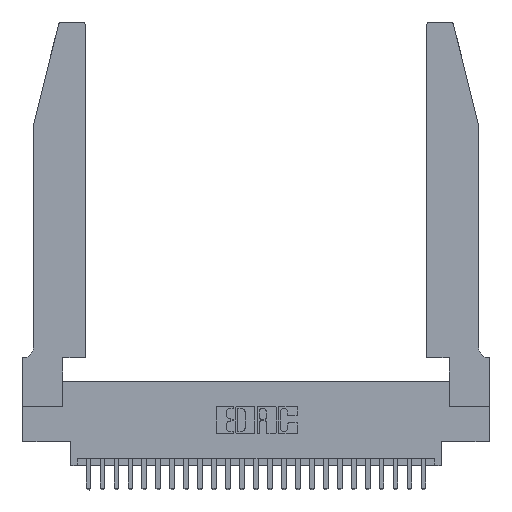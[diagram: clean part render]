
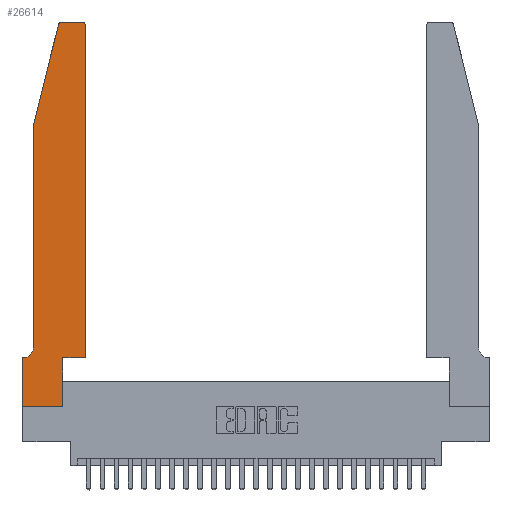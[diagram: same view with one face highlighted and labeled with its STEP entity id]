
A CAD part, top view. The second image highlights one B-rep face of the part: STEP entity #26614.
In plain terms, the highlighted planar face has unit normal (0, 0, 1).
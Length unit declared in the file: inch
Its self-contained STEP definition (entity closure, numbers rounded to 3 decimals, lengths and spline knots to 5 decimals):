
#441 = DIRECTION ( 'NONE',  ( 0., 1., 0. ) ) ;
#812 = ORIENTED_EDGE ( 'NONE', *, *, #13070, .T. ) ;
#826 = CARTESIAN_POINT ( 'NONE',  ( 0.4505, 0.35, 0.37 ) ) ;
#1180 = CIRCLE ( 'NONE', #20505, 0.07 ) ;
#1623 = DIRECTION ( 'NONE',  ( -0.239, -0.971, 0. ) ) ;
#1858 = EDGE_CURVE ( 'NONE', #19033, #4692, #2163, .T. ) ;
#2163 = LINE ( 'NONE', #8192, #22024 ) ;
#2244 = DIRECTION ( 'NONE',  ( 0., 0., 1. ) ) ;
#3155 = DIRECTION ( 'NONE',  ( 1., 0., 0. ) ) ;
#3374 = CARTESIAN_POINT ( 'NONE',  ( 0., 0.35, 0.37 ) ) ;
#3847 = ORIENTED_EDGE ( 'NONE', *, *, #15759, .T. ) ;
#3925 = EDGE_CURVE ( 'NONE', #5902, #19767, #11113, .T. ) ;
#4187 = CARTESIAN_POINT ( 'NONE',  ( 0.4505, 0.35, 0.37 ) ) ;
#4507 = VECTOR ( 'NONE', #7027, 39.37008 ) ;
#4586 = CARTESIAN_POINT ( 'NONE',  ( 0.2865, 0.35, 0.37 ) ) ;
#4692 = VERTEX_POINT ( 'NONE', #15383 ) ;
#5426 = CARTESIAN_POINT ( 'NONE',  ( 0., 0.35, 0.37 ) ) ;
#5545 = VERTEX_POINT ( 'NONE', #8538 ) ;
#5902 = VERTEX_POINT ( 'NONE', #25741 ) ;
#6135 = ORIENTED_EDGE ( 'NONE', *, *, #3925, .T. ) ;
#6289 = CARTESIAN_POINT ( 'NONE',  ( 0.284, 2.72, 0.37 ) ) ;
#6410 = EDGE_CURVE ( 'NONE', #12512, #19033, #11972, .T. ) ;
#6717 = VECTOR ( 'NONE', #21483, 39.37008 ) ;
#7027 = DIRECTION ( 'NONE',  ( 1., 0., 0. ) ) ;
#7376 = CIRCLE ( 'NONE', #15077, 0.03 ) ;
#7941 = CARTESIAN_POINT ( 'NONE',  ( 0.0755, 2., 0.37 ) ) ;
#7953 = VERTEX_POINT ( 'NONE', #15384 ) ;
#7997 = LINE ( 'NONE', #7941, #19749 ) ;
#8192 = CARTESIAN_POINT ( 'NONE',  ( 0., 0., 0.37 ) ) ;
#8538 = CARTESIAN_POINT ( 'NONE',  ( 0.4505, 2.72, 0.37 ) ) ;
#8663 = DIRECTION ( 'NONE',  ( 0., 0., -1. ) ) ;
#8692 = VECTOR ( 'NONE', #3155, 39.37008 ) ;
#9043 = VECTOR ( 'NONE', #12936, 39.37008 ) ;
#9156 = FACE_OUTER_BOUND ( 'NONE', #16446, .T. ) ;
#9232 = ORIENTED_EDGE ( 'NONE', *, *, #6410, .T. ) ;
#9514 = VERTEX_POINT ( 'NONE', #9903 ) ;
#9901 = ORIENTED_EDGE ( 'NONE', *, *, #1858, .T. ) ;
#9903 = CARTESIAN_POINT ( 'NONE',  ( 0.2865, 0., 0.37 ) ) ;
#10303 = DIRECTION ( 'NONE',  ( 0., -1., 0. ) ) ;
#10632 = VERTEX_POINT ( 'NONE', #23169 ) ;
#10888 = EDGE_CURVE ( 'NONE', #9514, #26902, #20522, .T. ) ;
#10955 = CARTESIAN_POINT ( 'NONE',  ( 0.2605, 2.75, 0.37 ) ) ;
#11060 = VECTOR ( 'NONE', #441, 39.37008 ) ;
#11113 = LINE ( 'NONE', #10955, #12097 ) ;
#11406 = ORIENTED_EDGE ( 'NONE', *, *, #16153, .T. ) ;
#11458 = VERTEX_POINT ( 'NONE', #21474 ) ;
#11972 = LINE ( 'NONE', #23353, #9043 ) ;
#11974 = LINE ( 'NONE', #21814, #8692 ) ;
#12097 = VECTOR ( 'NONE', #21168, 39.37008 ) ;
#12181 = EDGE_CURVE ( 'NONE', #10632, #11458, #21130, .T. ) ;
#12512 = VERTEX_POINT ( 'NONE', #17127 ) ;
#12936 = DIRECTION ( 'NONE',  ( -1., 0., 0. ) ) ;
#13070 = EDGE_CURVE ( 'NONE', #20444, #5545, #23710, .T. ) ;
#13475 = EDGE_CURVE ( 'NONE', #11458, #7953, #7997, .T. ) ;
#13948 = DIRECTION ( 'NONE',  ( 0., 0., 1. ) ) ;
#14024 = CARTESIAN_POINT ( 'NONE',  ( 0.0755, 2., 0.37 ) ) ;
#14582 = CIRCLE ( 'NONE', #26066, 0.03 ) ;
#14740 = DIRECTION ( 'NONE',  ( 1., 0., 0. ) ) ;
#15077 = AXIS2_PLACEMENT_3D ( 'NONE', #6289, #2244, #14740 ) ;
#15281 = VECTOR ( 'NONE', #1623, 39.37008 ) ;
#15383 = CARTESIAN_POINT ( 'NONE',  ( 0., 0., 0.37 ) ) ;
#15384 = CARTESIAN_POINT ( 'NONE',  ( 0.0755, 0.42, 0.37 ) ) ;
#15528 = EDGE_CURVE ( 'NONE', #5545, #5902, #14582, .T. ) ;
#15668 = EDGE_CURVE ( 'NONE', #4692, #9514, #11974, .T. ) ;
#15717 = ORIENTED_EDGE ( 'NONE', *, *, #10888, .T. ) ;
#15759 = EDGE_CURVE ( 'NONE', #26902, #20444, #16299, .T. ) ;
#15888 = PLANE ( 'NONE',  #17153 ) ;
#15909 = CARTESIAN_POINT ( 'NONE',  ( 0.4505, 0.35, 0.37 ) ) ;
#16153 = EDGE_CURVE ( 'NONE', #19767, #10632, #7376, .T. ) ;
#16299 = LINE ( 'NONE', #826, #4507 ) ;
#16446 = EDGE_LOOP ( 'NONE', ( #6135, #11406, #21901, #20417, #22272, #9232, #9901, #24777, #15717, #3847, #812, #17753 ) ) ;
#16972 = CARTESIAN_POINT ( 'NONE',  ( 0.0055, 0.42, 0.37 ) ) ;
#17127 = CARTESIAN_POINT ( 'NONE',  ( 0.0055, 0.35, 0.37 ) ) ;
#17153 = AXIS2_PLACEMENT_3D ( 'NONE', #5426, #13948, #24194 ) ;
#17630 = EDGE_CURVE ( 'NONE', #7953, #12512, #1180, .T. ) ;
#17753 = ORIENTED_EDGE ( 'NONE', *, *, #15528, .T. ) ;
#18966 = CARTESIAN_POINT ( 'NONE',  ( 0.2865, 0.35, 0.37 ) ) ;
#19033 = VERTEX_POINT ( 'NONE', #3374 ) ;
#19332 = DIRECTION ( 'NONE',  ( 0., 0., 1. ) ) ;
#19337 = DIRECTION ( 'NONE',  ( -1., 0., 0. ) ) ;
#19749 = VECTOR ( 'NONE', #22570, 39.37008 ) ;
#19767 = VERTEX_POINT ( 'NONE', #24330 ) ;
#20417 = ORIENTED_EDGE ( 'NONE', *, *, #13475, .T. ) ;
#20444 = VERTEX_POINT ( 'NONE', #15909 ) ;
#20505 = AXIS2_PLACEMENT_3D ( 'NONE', #16972, #8663, #19337 ) ;
#20522 = LINE ( 'NONE', #4586, #11060 ) ;
#21130 = LINE ( 'NONE', #14024, #15281 ) ;
#21168 = DIRECTION ( 'NONE',  ( -1., 0., 0. ) ) ;
#21345 = DIRECTION ( 'NONE',  ( 1., 0., 0. ) ) ;
#21474 = CARTESIAN_POINT ( 'NONE',  ( 0.0755, 2., 0.37 ) ) ;
#21483 = DIRECTION ( 'NONE',  ( 0., 1., 0. ) ) ;
#21814 = CARTESIAN_POINT ( 'NONE',  ( 0., 0., 0.37 ) ) ;
#21901 = ORIENTED_EDGE ( 'NONE', *, *, #12181, .T. ) ;
#22024 = VECTOR ( 'NONE', #10303, 39.37008 ) ;
#22272 = ORIENTED_EDGE ( 'NONE', *, *, #17630, .T. ) ;
#22570 = DIRECTION ( 'NONE',  ( 0., -1., 0. ) ) ;
#23169 = CARTESIAN_POINT ( 'NONE',  ( 0.25487, 2.72718, 0.37 ) ) ;
#23353 = CARTESIAN_POINT ( 'NONE',  ( 0.0755, 0.35, 0.37 ) ) ;
#23454 = CARTESIAN_POINT ( 'NONE',  ( 0.4205, 2.72, 0.37 ) ) ;
#23710 = LINE ( 'NONE', #4187, #6717 ) ;
#24194 = DIRECTION ( 'NONE',  ( 1., 0., 0. ) ) ;
#24330 = CARTESIAN_POINT ( 'NONE',  ( 0.284, 2.75, 0.37 ) ) ;
#24777 = ORIENTED_EDGE ( 'NONE', *, *, #15668, .T. ) ;
#25741 = CARTESIAN_POINT ( 'NONE',  ( 0.4205, 2.75, 0.37 ) ) ;
#26066 = AXIS2_PLACEMENT_3D ( 'NONE', #23454, #19332, #21345 ) ;
#26614 = ADVANCED_FACE ( 'NONE', ( #9156 ), #15888, .T. ) ;
#26902 = VERTEX_POINT ( 'NONE', #18966 ) ;
